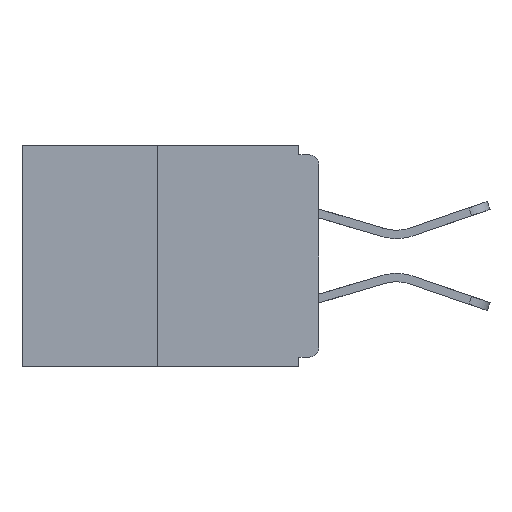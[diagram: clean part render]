
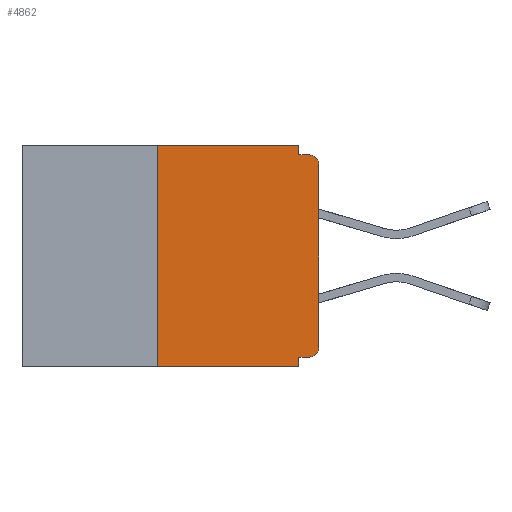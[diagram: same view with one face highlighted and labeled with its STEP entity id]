
A CAD part, left-side view. The second image highlights one B-rep face of the part: STEP entity #4862.
In plain terms, the highlighted planar face has unit normal (-1, 0, 0).
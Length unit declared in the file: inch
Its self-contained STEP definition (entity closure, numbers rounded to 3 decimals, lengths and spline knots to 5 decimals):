
#295 = ORIENTED_EDGE ( 'NONE', *, *, #5636, .F. ) ;
#429 = ORIENTED_EDGE ( 'NONE', *, *, #2896, .F. ) ;
#564 = VECTOR ( 'NONE', #6514, 39.37008 ) ;
#777 = CARTESIAN_POINT ( 'NONE',  ( 0., 0.031, 0. ) ) ;
#812 = CARTESIAN_POINT ( 'NONE',  ( 0., 0., -0.328 ) ) ;
#917 = LINE ( 'NONE', #6102, #2147 ) ;
#1107 = VECTOR ( 'NONE', #14505, 39.37008 ) ;
#1936 = ORIENTED_EDGE ( 'NONE', *, *, #11094, .F. ) ;
#2041 = VERTEX_POINT ( 'NONE', #4029 ) ;
#2049 = CARTESIAN_POINT ( 'NONE',  ( 0., 0.031, -0.015 ) ) ;
#2147 = VECTOR ( 'NONE', #14351, 39.37008 ) ;
#2229 = CARTESIAN_POINT ( 'NONE',  ( 0., 0.015, -0.328 ) ) ;
#2496 = EDGE_CURVE ( 'NONE', #9568, #3287, #10038, .T. ) ;
#2514 = EDGE_CURVE ( 'NONE', #14178, #2041, #13047, .T. ) ;
#2613 = ORIENTED_EDGE ( 'NONE', *, *, #3394, .F. ) ;
#2732 = CARTESIAN_POINT ( 'NONE',  ( 0., 0.25, -0.343 ) ) ;
#2896 = EDGE_CURVE ( 'NONE', #12614, #5518, #3751, .T. ) ;
#2906 = DIRECTION ( 'NONE',  ( 0., 0., -1. ) ) ;
#3010 = CARTESIAN_POINT ( 'NONE',  ( 0., 0.46, 0. ) ) ;
#3168 = CARTESIAN_POINT ( 'NONE',  ( 0., 0.031, -0.343 ) ) ;
#3271 = LINE ( 'NONE', #812, #12299 ) ;
#3287 = VERTEX_POINT ( 'NONE', #4917 ) ;
#3304 = EDGE_CURVE ( 'NONE', #12039, #9484, #917, .T. ) ;
#3394 = EDGE_CURVE ( 'NONE', #8373, #12614, #10199, .T. ) ;
#3751 = LINE ( 'NONE', #11926, #564 ) ;
#3858 = AXIS2_PLACEMENT_3D ( 'NONE', #5162, #6508, #2906 ) ;
#4029 = CARTESIAN_POINT ( 'NONE',  ( 0., 0.015, -0.015 ) ) ;
#4042 = CARTESIAN_POINT ( 'NONE',  ( 0., 0.46, 0. ) ) ;
#4167 = DIRECTION ( 'NONE',  ( 0., 0., -1. ) ) ;
#4862 = ADVANCED_FACE ( 'NONE', ( #8378 ), #10023, .F. ) ;
#4917 = CARTESIAN_POINT ( 'NONE',  ( 0., 0., -0.313 ) ) ;
#5038 = ORIENTED_EDGE ( 'NONE', *, *, #3304, .F. ) ;
#5107 = VECTOR ( 'NONE', #11634, 39.37008 ) ;
#5162 = CARTESIAN_POINT ( 'NONE',  ( 0., 0.015, -0.313 ) ) ;
#5484 = AXIS2_PLACEMENT_3D ( 'NONE', #6355, #14331, #4167 ) ;
#5518 = VERTEX_POINT ( 'NONE', #2049 ) ;
#5570 = DIRECTION ( 'NONE',  ( 0., -1., 0. ) ) ;
#5636 = EDGE_CURVE ( 'NONE', #5518, #2041, #9413, .T. ) ;
#5881 = EDGE_CURVE ( 'NONE', #3287, #14178, #13335, .T. ) ;
#5921 = ORIENTED_EDGE ( 'NONE', *, *, #10536, .T. ) ;
#6102 = CARTESIAN_POINT ( 'NONE',  ( 0., 0.031, -0.343 ) ) ;
#6189 = DIRECTION ( 'NONE',  ( 0., 0., 1. ) ) ;
#6354 = VECTOR ( 'NONE', #5570, 39.37008 ) ;
#6355 = CARTESIAN_POINT ( 'NONE',  ( 0., 0.015, -0.03 ) ) ;
#6373 = CARTESIAN_POINT ( 'NONE',  ( 0., 0.46, -0.343 ) ) ;
#6508 = DIRECTION ( 'NONE',  ( -1., 0., 0. ) ) ;
#6514 = DIRECTION ( 'NONE',  ( 0., 0., -1. ) ) ;
#7140 = ORIENTED_EDGE ( 'NONE', *, *, #2514, .T. ) ;
#7758 = DIRECTION ( 'NONE',  ( 0., 0., -1. ) ) ;
#7842 = VECTOR ( 'NONE', #13172, 39.37008 ) ;
#7923 = CARTESIAN_POINT ( 'NONE',  ( 0., 0.031, -0.328 ) ) ;
#8373 = VERTEX_POINT ( 'NONE', #14661 ) ;
#8378 = FACE_OUTER_BOUND ( 'NONE', #8866, .T. ) ;
#8604 = CARTESIAN_POINT ( 'NONE',  ( 0., 0., 0. ) ) ;
#8866 = EDGE_LOOP ( 'NONE', ( #2613, #10940, #5921, #5038, #1936, #13097, #9270, #7140, #295, #429 ) ) ;
#8883 = LINE ( 'NONE', #10283, #5107 ) ;
#9128 = CARTESIAN_POINT ( 'NONE',  ( 0., 0., -0.015 ) ) ;
#9270 = ORIENTED_EDGE ( 'NONE', *, *, #5881, .T. ) ;
#9413 = LINE ( 'NONE', #9128, #6354 ) ;
#9484 = VERTEX_POINT ( 'NONE', #3168 ) ;
#9568 = VERTEX_POINT ( 'NONE', #2229 ) ;
#9945 = DIRECTION ( 'NONE',  ( 0., 1., 0. ) ) ;
#10023 = PLANE ( 'NONE',  #10599 ) ;
#10038 = CIRCLE ( 'NONE', #3858, 0.015 ) ;
#10199 = LINE ( 'NONE', #4042, #1107 ) ;
#10283 = CARTESIAN_POINT ( 'NONE',  ( 0., 0.25, 0. ) ) ;
#10536 = EDGE_CURVE ( 'NONE', #13462, #9484, #12682, .T. ) ;
#10599 = AXIS2_PLACEMENT_3D ( 'NONE', #3010, #11033, #7758 ) ;
#10940 = ORIENTED_EDGE ( 'NONE', *, *, #12128, .F. ) ;
#11033 = DIRECTION ( 'NONE',  ( 1., 0., 0. ) ) ;
#11094 = EDGE_CURVE ( 'NONE', #9568, #12039, #3271, .T. ) ;
#11634 = DIRECTION ( 'NONE',  ( 0., 0., 1. ) ) ;
#11926 = CARTESIAN_POINT ( 'NONE',  ( 0., 0.031, 0. ) ) ;
#12039 = VERTEX_POINT ( 'NONE', #7923 ) ;
#12128 = EDGE_CURVE ( 'NONE', #13462, #8373, #8883, .T. ) ;
#12299 = VECTOR ( 'NONE', #9945, 39.37008 ) ;
#12614 = VERTEX_POINT ( 'NONE', #777 ) ;
#12630 = VECTOR ( 'NONE', #6189, 39.37008 ) ;
#12682 = LINE ( 'NONE', #6373, #7842 ) ;
#12893 = CARTESIAN_POINT ( 'NONE',  ( 0., 0., -0.03 ) ) ;
#13047 = CIRCLE ( 'NONE', #5484, 0.015 ) ;
#13097 = ORIENTED_EDGE ( 'NONE', *, *, #2496, .T. ) ;
#13172 = DIRECTION ( 'NONE',  ( 0., -1., 0. ) ) ;
#13335 = LINE ( 'NONE', #8604, #12630 ) ;
#13462 = VERTEX_POINT ( 'NONE', #2732 ) ;
#14178 = VERTEX_POINT ( 'NONE', #12893 ) ;
#14331 = DIRECTION ( 'NONE',  ( -1., 0., 0. ) ) ;
#14351 = DIRECTION ( 'NONE',  ( 0., 0., -1. ) ) ;
#14505 = DIRECTION ( 'NONE',  ( 0., -1., 0. ) ) ;
#14661 = CARTESIAN_POINT ( 'NONE',  ( 0., 0.25, 0. ) ) ;
